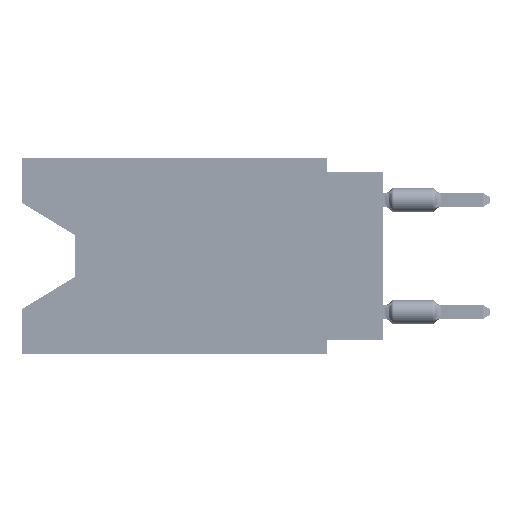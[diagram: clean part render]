
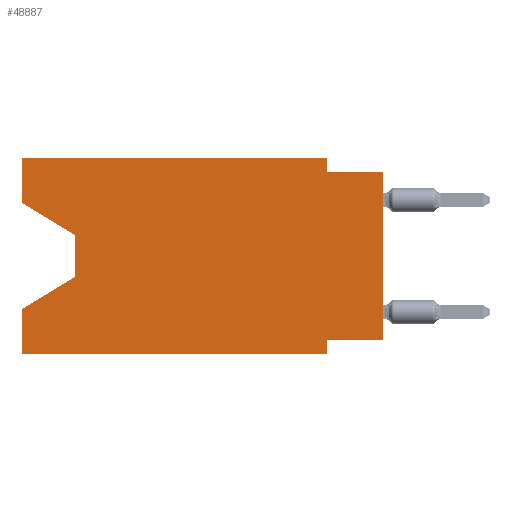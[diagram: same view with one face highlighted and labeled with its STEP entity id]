
A CAD part, left-side view. The second image highlights one B-rep face of the part: STEP entity #48887.
In plain terms, the highlighted planar face has unit normal (-1, 0, 0).
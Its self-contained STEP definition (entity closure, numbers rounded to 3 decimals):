
#134 = VERTEX_POINT ( 'NONE', #55718 ) ;
#1176 = ORIENTED_EDGE ( 'NONE', *, *, #59688, .T. ) ;
#1336 = ORIENTED_EDGE ( 'NONE', *, *, #3000, .F. ) ;
#1778 = VERTEX_POINT ( 'NONE', #26998 ) ;
#1832 = CARTESIAN_POINT ( 'NONE',  ( 0., 16.383, 0. ) ) ;
#2449 = CARTESIAN_POINT ( 'NONE',  ( 0., 0., 0. ) ) ;
#3000 = EDGE_CURVE ( 'NONE', #24923, #4580, #27962, .T. ) ;
#4282 = LINE ( 'NONE', #46617, #52445 ) ;
#4460 = LINE ( 'NONE', #8723, #50543 ) ;
#4580 = VERTEX_POINT ( 'NONE', #52998 ) ;
#5746 = LINE ( 'NONE', #25200, #34032 ) ;
#5768 = CARTESIAN_POINT ( 'NONE',  ( 0., 13.97, -5.385 ) ) ;
#5790 = DIRECTION ( 'NONE',  ( 0., 0., 1. ) ) ;
#5965 = EDGE_CURVE ( 'NONE', #45903, #16232, #37137, .T. ) ;
#7568 = ORIENTED_EDGE ( 'NONE', *, *, #11653, .F. ) ;
#8400 = CARTESIAN_POINT ( 'NONE',  ( 0., 2.54, 0. ) ) ;
#8723 = CARTESIAN_POINT ( 'NONE',  ( 0., 13.97, -3.505 ) ) ;
#8790 = LINE ( 'NONE', #23416, #13462 ) ;
#10870 = VERTEX_POINT ( 'NONE', #23844 ) ;
#11238 = CARTESIAN_POINT ( 'NONE',  ( 0., 16.383, 0. ) ) ;
#11653 = EDGE_CURVE ( 'NONE', #10870, #16232, #34113, .T. ) ;
#12341 = CARTESIAN_POINT ( 'NONE',  ( 0., 2.54, -0.635 ) ) ;
#13462 = VECTOR ( 'NONE', #55729, 1000. ) ;
#14449 = EDGE_LOOP ( 'NONE', ( #35421, #41133, #38035, #7568, #1176, #29498, #47705, #42942, #19390, #59149, #1336, #15550 ) ) ;
#14842 = DIRECTION ( 'NONE',  ( 0., -1., 0. ) ) ;
#15421 = VERTEX_POINT ( 'NONE', #12341 ) ;
#15550 = ORIENTED_EDGE ( 'NONE', *, *, #50466, .F. ) ;
#16232 = VERTEX_POINT ( 'NONE', #42990 ) ;
#18588 = CARTESIAN_POINT ( 'NONE',  ( 0., 0., -0.635 ) ) ;
#19390 = ORIENTED_EDGE ( 'NONE', *, *, #25126, .F. ) ;
#19795 = CARTESIAN_POINT ( 'NONE',  ( 0., 16.383, 0. ) ) ;
#19815 = FACE_OUTER_BOUND ( 'NONE', #14449, .T. ) ;
#20353 = VERTEX_POINT ( 'NONE', #27716 ) ;
#21198 = AXIS2_PLACEMENT_3D ( 'NONE', #1832, #56692, #42953 ) ;
#21205 = VECTOR ( 'NONE', #47892, 1000. ) ;
#21963 = DIRECTION ( 'NONE',  ( 0., -1., 0. ) ) ;
#23416 = CARTESIAN_POINT ( 'NONE',  ( 0., 0., -8.255 ) ) ;
#23487 = EDGE_CURVE ( 'NONE', #4580, #15421, #53824, .T. ) ;
#23642 = DIRECTION ( 'NONE',  ( 0., 0., -1. ) ) ;
#23844 = CARTESIAN_POINT ( 'NONE',  ( 0., 16.383, -8.89 ) ) ;
#24077 = VERTEX_POINT ( 'NONE', #59825 ) ;
#24491 = VECTOR ( 'NONE', #14842, 1000. ) ;
#24923 = VERTEX_POINT ( 'NONE', #11238 ) ;
#25126 = EDGE_CURVE ( 'NONE', #15421, #134, #32007, .T. ) ;
#25200 = CARTESIAN_POINT ( 'NONE',  ( 0., 16.383, 0. ) ) ;
#25578 = LINE ( 'NONE', #2449, #31465 ) ;
#26647 = VERTEX_POINT ( 'NONE', #27192 ) ;
#26998 = CARTESIAN_POINT ( 'NONE',  ( 0., 16.383, -2.038 ) ) ;
#27192 = CARTESIAN_POINT ( 'NONE',  ( 0., 13.97, -3.505 ) ) ;
#27716 = CARTESIAN_POINT ( 'NONE',  ( 0., 2.54, -8.255 ) ) ;
#27962 = LINE ( 'NONE', #33140, #24491 ) ;
#28741 = DIRECTION ( 'NONE',  ( 0., 0., 1. ) ) ;
#29498 = ORIENTED_EDGE ( 'NONE', *, *, #47106, .F. ) ;
#31105 = VECTOR ( 'NONE', #21963, 1000. ) ;
#31465 = VECTOR ( 'NONE', #28741, 1000. ) ;
#32007 = LINE ( 'NONE', #18588, #31105 ) ;
#32575 = CARTESIAN_POINT ( 'NONE',  ( 0., 13.97, -5.385 ) ) ;
#32863 = VECTOR ( 'NONE', #54456, 1000. ) ;
#33140 = CARTESIAN_POINT ( 'NONE',  ( 0., 16.383, 0. ) ) ;
#34032 = VECTOR ( 'NONE', #39218, 1000. ) ;
#34113 = LINE ( 'NONE', #19795, #43612 ) ;
#35421 = ORIENTED_EDGE ( 'NONE', *, *, #37946, .T. ) ;
#35567 = LINE ( 'NONE', #54161, #32863 ) ;
#35911 = CARTESIAN_POINT ( 'NONE',  ( 0., 2.54, -8.89 ) ) ;
#37137 = LINE ( 'NONE', #32575, #43149 ) ;
#37617 = VECTOR ( 'NONE', #39788, 1000. ) ;
#37946 = EDGE_CURVE ( 'NONE', #1778, #26647, #35567, .T. ) ;
#38035 = ORIENTED_EDGE ( 'NONE', *, *, #5965, .T. ) ;
#38521 = EDGE_CURVE ( 'NONE', #24077, #134, #25578, .T. ) ;
#39218 = DIRECTION ( 'NONE',  ( 0., 0., 1. ) ) ;
#39788 = DIRECTION ( 'NONE',  ( 0., 0., -1. ) ) ;
#41133 = ORIENTED_EDGE ( 'NONE', *, *, #50660, .T. ) ;
#42561 = VERTEX_POINT ( 'NONE', #35911 ) ;
#42942 = ORIENTED_EDGE ( 'NONE', *, *, #38521, .T. ) ;
#42953 = DIRECTION ( 'NONE',  ( 0., 0., -1. ) ) ;
#42990 = CARTESIAN_POINT ( 'NONE',  ( 0., 16.383, -6.852 ) ) ;
#43149 = VECTOR ( 'NONE', #51130, 1000. ) ;
#43566 = PLANE ( 'NONE',  #21198 ) ;
#43612 = VECTOR ( 'NONE', #5790, 1000. ) ;
#45903 = VERTEX_POINT ( 'NONE', #5768 ) ;
#46617 = CARTESIAN_POINT ( 'NONE',  ( 0., 16.383, -8.89 ) ) ;
#47106 = EDGE_CURVE ( 'NONE', #20353, #42561, #53071, .T. ) ;
#47705 = ORIENTED_EDGE ( 'NONE', *, *, #49117, .F. ) ;
#47892 = DIRECTION ( 'NONE',  ( 0., 0., -1. ) ) ;
#48887 = ADVANCED_FACE ( 'NONE', ( #19815 ), #43566, .F. ) ;
#49117 = EDGE_CURVE ( 'NONE', #24077, #20353, #8790, .T. ) ;
#50466 = EDGE_CURVE ( 'NONE', #1778, #24923, #5746, .T. ) ;
#50543 = VECTOR ( 'NONE', #23642, 1000. ) ;
#50660 = EDGE_CURVE ( 'NONE', #26647, #45903, #4460, .T. ) ;
#51130 = DIRECTION ( 'NONE',  ( 0., 0.855, -0.519 ) ) ;
#52445 = VECTOR ( 'NONE', #59733, 1000. ) ;
#52998 = CARTESIAN_POINT ( 'NONE',  ( 0., 2.54, 0. ) ) ;
#53071 = LINE ( 'NONE', #57651, #21205 ) ;
#53824 = LINE ( 'NONE', #8400, #37617 ) ;
#54161 = CARTESIAN_POINT ( 'NONE',  ( 0., 16.383, -2.038 ) ) ;
#54456 = DIRECTION ( 'NONE',  ( 0., -0.855, -0.519 ) ) ;
#55718 = CARTESIAN_POINT ( 'NONE',  ( 0., 0., -0.635 ) ) ;
#55729 = DIRECTION ( 'NONE',  ( 0., 1., 0. ) ) ;
#56692 = DIRECTION ( 'NONE',  ( 1., 0., 0. ) ) ;
#57651 = CARTESIAN_POINT ( 'NONE',  ( 0., 2.54, -8.89 ) ) ;
#59149 = ORIENTED_EDGE ( 'NONE', *, *, #23487, .F. ) ;
#59688 = EDGE_CURVE ( 'NONE', #10870, #42561, #4282, .T. ) ;
#59733 = DIRECTION ( 'NONE',  ( 0., -1., 0. ) ) ;
#59825 = CARTESIAN_POINT ( 'NONE',  ( 0., 0., -8.255 ) ) ;
